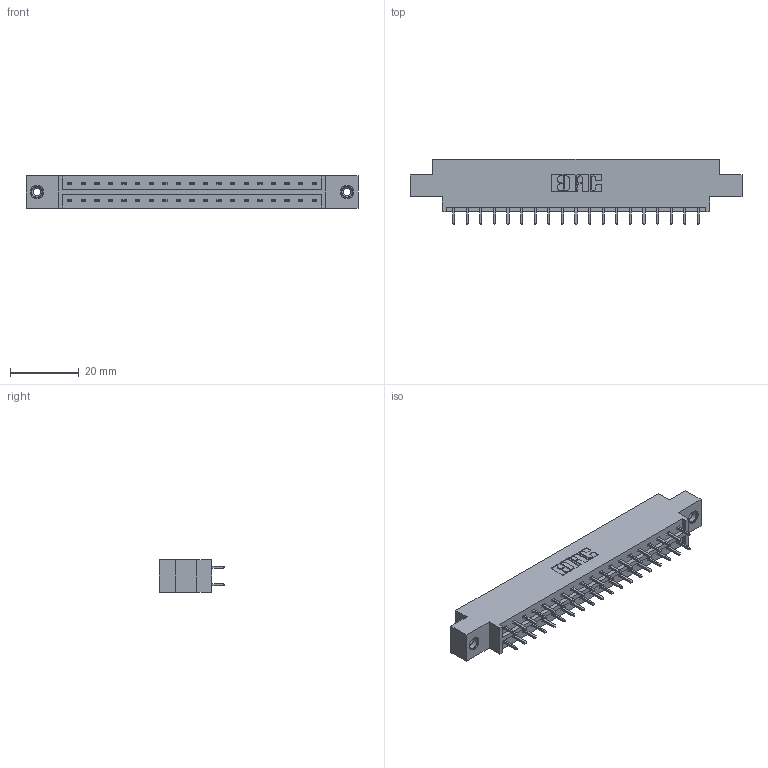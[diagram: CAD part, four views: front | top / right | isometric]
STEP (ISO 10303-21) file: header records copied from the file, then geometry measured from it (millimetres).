
FILE_DESCRIPTION (( 'STEP AP203' ), '1' );
FILE_NAME ('833-038-521-808.STEP', '2020-06-03T06:46:41', ( '' ), ( '' ), 'SwSTEP 2.0', 'SolidWorks 2020', '' );
FILE_SCHEMA (( 'CONFIG_CONTROL_DESIGN' ));
Length unit declared in the file: inch
Products named in the file (4): 345-292-001_345-293-121; 833 Part_Offset - .156 Dia - TI; 345-250-001_345-250-003-102; 833-038-521-808
Assembly tree (41 placements, depth 2):
  833-038-521-808
    833 Part_Offset - .156 Dia - TI
    345-292-001_345-293-121  x38
    345-250-001_345-250-003-102  x2
Bounding box: 96.82 x 19.06 x 9.4 mm (x, y, z)
Volume: 9420.3 mm3; surface area: 11023.3 mm2
Topology: 41 solids, 41 shells, 2154 faces, 6349 edges, 4174 vertices
Faces by surface type: plane 1474, cylinder 664, cone 12, torus 4
Entity records: 16534 total; most frequent: CARTESIAN_POINT 2753, ORIENTED_EDGE 2682, DIRECTION 2423, EDGE_CURVE 1341, VECTOR 1193, LINE 1193, VERTEX_POINT 888, AXIS2_PLACEMENT_3D 615
